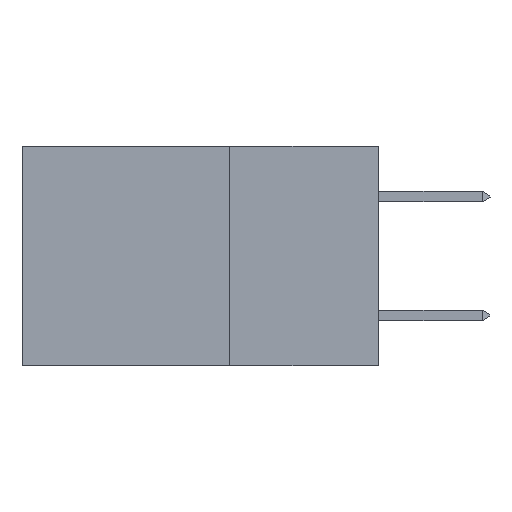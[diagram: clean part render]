
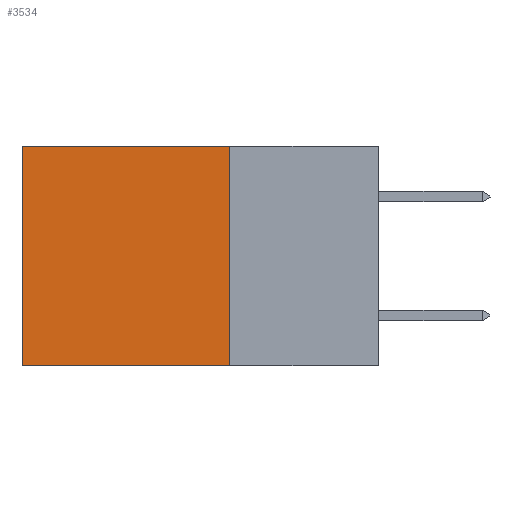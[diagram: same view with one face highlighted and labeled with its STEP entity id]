
A CAD part, left-side view. The second image highlights one B-rep face of the part: STEP entity #3534.
In plain terms, the highlighted planar face has unit normal (-1, 0, 0).
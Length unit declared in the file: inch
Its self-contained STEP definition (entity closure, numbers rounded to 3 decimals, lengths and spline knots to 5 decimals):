
#559 = VECTOR ( 'NONE', #16580, 39.37008 ) ;
#680 = ORIENTED_EDGE ( 'NONE', *, *, #6578, .T. ) ;
#998 = LINE ( 'NONE', #1272, #22754 ) ;
#1272 = CARTESIAN_POINT ( 'NONE',  ( 0.298, 0.25, -0.37 ) ) ;
#3331 = LINE ( 'NONE', #16159, #10402 ) ;
#3534 = ADVANCED_FACE ( 'NONE', ( #25518 ), #4833, .F. ) ;
#4502 = EDGE_LOOP ( 'NONE', ( #11176, #4630, #25325, #680 ) ) ;
#4597 = DIRECTION ( 'NONE',  ( 0., 0., -1. ) ) ;
#4630 = ORIENTED_EDGE ( 'NONE', *, *, #6313, .F. ) ;
#4833 = PLANE ( 'NONE',  #19679 ) ;
#5690 = LINE ( 'NONE', #26554, #26139 ) ;
#6313 = EDGE_CURVE ( 'NONE', #23995, #15026, #998, .T. ) ;
#6578 = EDGE_CURVE ( 'NONE', #24819, #16662, #32220, .T. ) ;
#7710 = CARTESIAN_POINT ( 'NONE',  ( 0.298, 0.25, -0.37 ) ) ;
#10362 = CARTESIAN_POINT ( 'NONE',  ( 0.298, 0.6, 0. ) ) ;
#10402 = VECTOR ( 'NONE', #21716, 39.37008 ) ;
#10571 = DIRECTION ( 'NONE',  ( 0., 0., -1. ) ) ;
#11124 = CARTESIAN_POINT ( 'NONE',  ( 0.298, 0.25, 0. ) ) ;
#11176 = ORIENTED_EDGE ( 'NONE', *, *, #24488, .T. ) ;
#15026 = VERTEX_POINT ( 'NONE', #27341 ) ;
#16159 = CARTESIAN_POINT ( 'NONE',  ( 0.298, 0.6, 0. ) ) ;
#16580 = DIRECTION ( 'NONE',  ( 0., 1., 0. ) ) ;
#16662 = VERTEX_POINT ( 'NONE', #10362 ) ;
#19679 = AXIS2_PLACEMENT_3D ( 'NONE', #23502, #31255, #4597 ) ;
#21716 = DIRECTION ( 'NONE',  ( 0., 0., -1. ) ) ;
#22410 = EDGE_CURVE ( 'NONE', #24819, #23995, #5690, .T. ) ;
#22754 = VECTOR ( 'NONE', #30880, 39.37008 ) ;
#23502 = CARTESIAN_POINT ( 'NONE',  ( 0.298, 0.25, 0. ) ) ;
#23995 = VERTEX_POINT ( 'NONE', #7710 ) ;
#24488 = EDGE_CURVE ( 'NONE', #16662, #15026, #3331, .T. ) ;
#24819 = VERTEX_POINT ( 'NONE', #28889 ) ;
#25325 = ORIENTED_EDGE ( 'NONE', *, *, #22410, .F. ) ;
#25518 = FACE_OUTER_BOUND ( 'NONE', #4502, .T. ) ;
#26139 = VECTOR ( 'NONE', #10571, 39.37008 ) ;
#26554 = CARTESIAN_POINT ( 'NONE',  ( 0.298, 0.25, 0. ) ) ;
#27341 = CARTESIAN_POINT ( 'NONE',  ( 0.298, 0.6, -0.37 ) ) ;
#28889 = CARTESIAN_POINT ( 'NONE',  ( 0.298, 0.25, 0. ) ) ;
#30880 = DIRECTION ( 'NONE',  ( 0., 1., 0. ) ) ;
#31255 = DIRECTION ( 'NONE',  ( 1., 0., 0. ) ) ;
#32220 = LINE ( 'NONE', #11124, #559 ) ;
